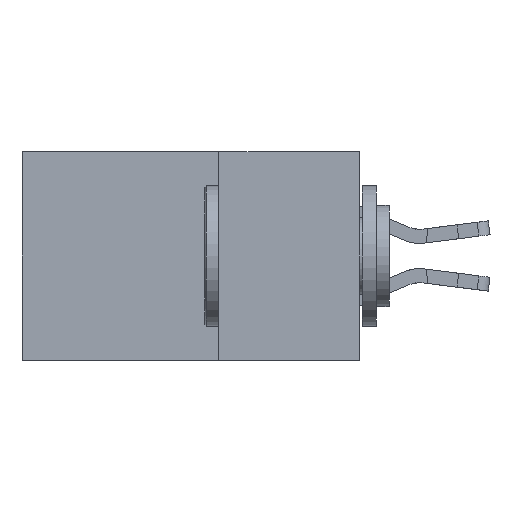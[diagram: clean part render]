
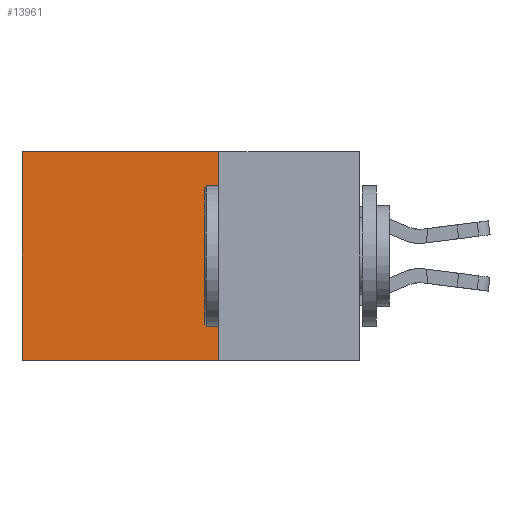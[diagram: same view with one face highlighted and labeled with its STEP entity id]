
A CAD part, left-side view. The second image highlights one B-rep face of the part: STEP entity #13961.
In plain terms, the highlighted planar face has unit normal (-1, 0, 0).
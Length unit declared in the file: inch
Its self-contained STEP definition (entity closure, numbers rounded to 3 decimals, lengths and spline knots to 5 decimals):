
#345 = ORIENTED_EDGE ( 'NONE', *, *, #8159, .F. ) ;
#772 = CARTESIAN_POINT ( 'NONE',  ( 0.2875, 0.6, 0. ) ) ;
#927 = DIRECTION ( 'NONE',  ( 0., 0., -1. ) ) ;
#2329 = CARTESIAN_POINT ( 'NONE',  ( 0.2875, 0.25, 0. ) ) ;
#2371 = VERTEX_POINT ( 'NONE', #13907 ) ;
#2739 = AXIS2_PLACEMENT_3D ( 'NONE', #2329, #11755, #3763 ) ;
#3380 = FACE_OUTER_BOUND ( 'NONE', #9264, .T. ) ;
#3542 = CARTESIAN_POINT ( 'NONE',  ( 0.2875, 0.25, 0. ) ) ;
#3763 = DIRECTION ( 'NONE',  ( 0., 0., -1. ) ) ;
#3982 = CARTESIAN_POINT ( 'NONE',  ( 0.2875, 0.6, -0.37 ) ) ;
#4014 = ORIENTED_EDGE ( 'NONE', *, *, #6916, .T. ) ;
#4197 = EDGE_CURVE ( 'NONE', #7954, #14835, #10512, .T. ) ;
#4507 = LINE ( 'NONE', #3542, #11174 ) ;
#4703 = LINE ( 'NONE', #10991, #10978 ) ;
#5659 = ORIENTED_EDGE ( 'NONE', *, *, #8434, .F. ) ;
#6916 = EDGE_CURVE ( 'NONE', #17391, #7954, #12686, .T. ) ;
#7954 = VERTEX_POINT ( 'NONE', #13865 ) ;
#8159 = EDGE_CURVE ( 'NONE', #17391, #2371, #4507, .T. ) ;
#8434 = EDGE_CURVE ( 'NONE', #2371, #14835, #4703, .T. ) ;
#9109 = PLANE ( 'NONE',  #2739 ) ;
#9195 = DIRECTION ( 'NONE',  ( 0., 1., 0. ) ) ;
#9264 = EDGE_LOOP ( 'NONE', ( #14461, #5659, #345, #4014 ) ) ;
#10512 = LINE ( 'NONE', #772, #13173 ) ;
#10978 = VECTOR ( 'NONE', #12310, 39.37008 ) ;
#10991 = CARTESIAN_POINT ( 'NONE',  ( 0.2875, 0.25, -0.37 ) ) ;
#11174 = VECTOR ( 'NONE', #14283, 39.37008 ) ;
#11755 = DIRECTION ( 'NONE',  ( 1., 0., 0. ) ) ;
#12266 = VECTOR ( 'NONE', #9195, 39.37008 ) ;
#12310 = DIRECTION ( 'NONE',  ( 0., 1., 0. ) ) ;
#12686 = LINE ( 'NONE', #15876, #12266 ) ;
#13173 = VECTOR ( 'NONE', #927, 39.37008 ) ;
#13865 = CARTESIAN_POINT ( 'NONE',  ( 0.2875, 0.6, 0. ) ) ;
#13907 = CARTESIAN_POINT ( 'NONE',  ( 0.2875, 0.25, -0.37 ) ) ;
#13961 = ADVANCED_FACE ( 'NONE', ( #3380 ), #9109, .F. ) ;
#14283 = DIRECTION ( 'NONE',  ( 0., 0., -1. ) ) ;
#14461 = ORIENTED_EDGE ( 'NONE', *, *, #4197, .T. ) ;
#14685 = CARTESIAN_POINT ( 'NONE',  ( 0.2875, 0.25, 0. ) ) ;
#14835 = VERTEX_POINT ( 'NONE', #3982 ) ;
#15876 = CARTESIAN_POINT ( 'NONE',  ( 0.2875, 0.25, 0. ) ) ;
#17391 = VERTEX_POINT ( 'NONE', #14685 ) ;
